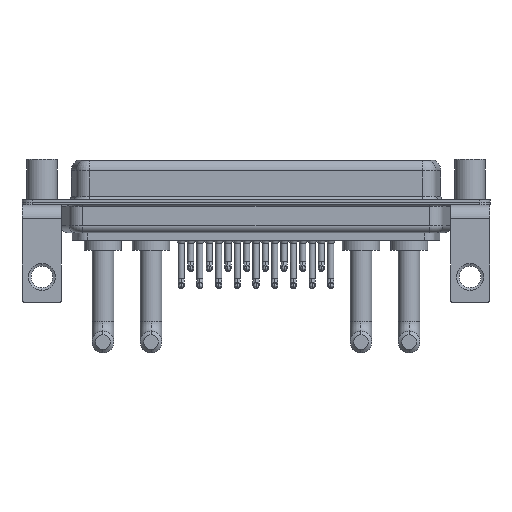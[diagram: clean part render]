
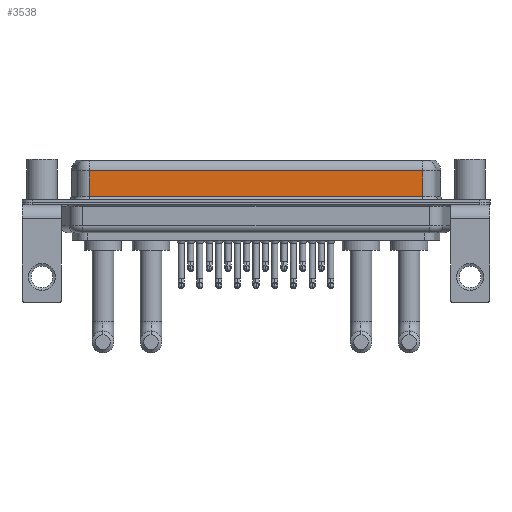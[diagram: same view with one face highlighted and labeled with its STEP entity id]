
A CAD part, front view. The second image highlights one B-rep face of the part: STEP entity #3538.
In plain terms, the highlighted planar face has unit normal (0, -1, 0).
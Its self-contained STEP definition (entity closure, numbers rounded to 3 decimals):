
#376 = EDGE_LOOP ( 'NONE', ( #6679, #21945, #9162, #3639 ) ) ;
#395 = VERTEX_POINT ( 'NONE', #7435 ) ;
#974 = EDGE_CURVE ( 'NONE', #16347, #395, #5908, .T. ) ;
#1144 = EDGE_CURVE ( 'NONE', #10558, #13360, #10732, .T. ) ;
#2607 = PLANE ( 'NONE',  #17131 ) ;
#3139 = DIRECTION ( 'NONE',  ( 0., 0., -1. ) ) ;
#3538 = ADVANCED_FACE ( 'NONE', ( #19623 ), #2607, .F. ) ;
#3639 = ORIENTED_EDGE ( 'NONE', *, *, #16577, .T. ) ;
#4252 = CARTESIAN_POINT ( 'NONE',  ( 56.462, -3.95, 0.9 ) ) ;
#4606 = DIRECTION ( 'NONE',  ( 0., 1., 0. ) ) ;
#4682 = VECTOR ( 'NONE', #22884, 1000. ) ;
#5908 = LINE ( 'NONE', #6158, #20643 ) ;
#6158 = CARTESIAN_POINT ( 'NONE',  ( 7.038, -3.95, 6.4 ) ) ;
#6443 = CARTESIAN_POINT ( 'NONE',  ( 56.462, -3.95, 0.9 ) ) ;
#6679 = ORIENTED_EDGE ( 'NONE', *, *, #1144, .F. ) ;
#7435 = CARTESIAN_POINT ( 'NONE',  ( 7.038, -3.95, 0.9 ) ) ;
#8152 = DIRECTION ( 'NONE',  ( 0., 0., -1. ) ) ;
#9162 = ORIENTED_EDGE ( 'NONE', *, *, #974, .T. ) ;
#10383 = CARTESIAN_POINT ( 'NONE',  ( 56.462, -3.95, 6.4 ) ) ;
#10558 = VERTEX_POINT ( 'NONE', #13505 ) ;
#10732 = LINE ( 'NONE', #10383, #15922 ) ;
#11147 = EDGE_CURVE ( 'NONE', #10558, #16347, #11613, .T. ) ;
#11613 = LINE ( 'NONE', #19058, #4682 ) ;
#11831 = DIRECTION ( 'NONE',  ( 1., 0., 0. ) ) ;
#12180 = DIRECTION ( 'NONE',  ( 0., 0., 1. ) ) ;
#13360 = VERTEX_POINT ( 'NONE', #6443 ) ;
#13505 = CARTESIAN_POINT ( 'NONE',  ( 56.462, -3.95, 4.65 ) ) ;
#15283 = CARTESIAN_POINT ( 'NONE',  ( 7.038, -3.95, 4.65 ) ) ;
#15916 = VECTOR ( 'NONE', #11831, 1000. ) ;
#15922 = VECTOR ( 'NONE', #3139, 1000. ) ;
#16347 = VERTEX_POINT ( 'NONE', #15283 ) ;
#16577 = EDGE_CURVE ( 'NONE', #395, #13360, #21244, .T. ) ;
#17131 = AXIS2_PLACEMENT_3D ( 'NONE', #21599, #4606, #12180 ) ;
#19058 = CARTESIAN_POINT ( 'NONE',  ( 56.462, -3.95, 4.65 ) ) ;
#19623 = FACE_OUTER_BOUND ( 'NONE', #376, .T. ) ;
#20643 = VECTOR ( 'NONE', #8152, 1000. ) ;
#21244 = LINE ( 'NONE', #4252, #15916 ) ;
#21599 = CARTESIAN_POINT ( 'NONE',  ( 56.462, -3.95, 6.4 ) ) ;
#21945 = ORIENTED_EDGE ( 'NONE', *, *, #11147, .T. ) ;
#22884 = DIRECTION ( 'NONE',  ( -1., 0., 0. ) ) ;
